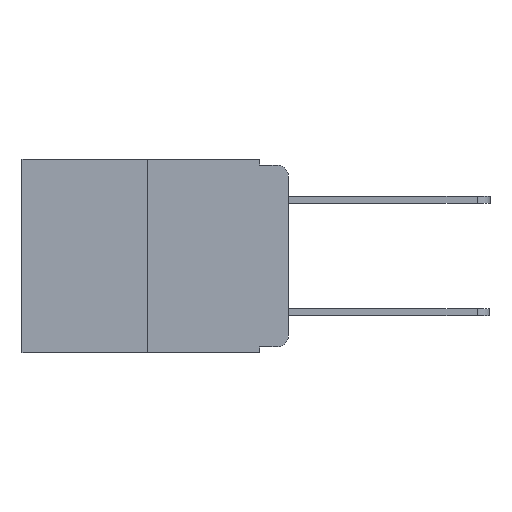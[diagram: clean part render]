
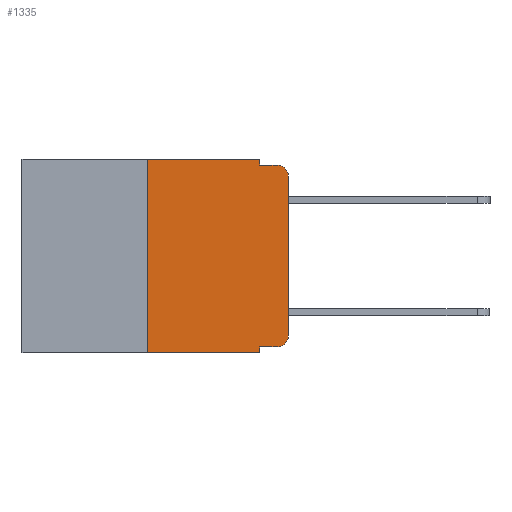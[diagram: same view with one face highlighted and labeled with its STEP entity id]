
A CAD part, left-side view. The second image highlights one B-rep face of the part: STEP entity #1335.
In plain terms, the highlighted planar face has unit normal (-1, 0, 0).
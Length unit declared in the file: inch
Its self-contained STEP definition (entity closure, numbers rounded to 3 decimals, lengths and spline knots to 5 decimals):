
#165 = VERTEX_POINT ( 'NONE', #10227 ) ;
#228 = EDGE_LOOP ( 'NONE', ( #6123, #8657, #6183, #6299, #9852, #9663, #3445, #1390, #520, #1811 ) ) ;
#249 = VECTOR ( 'NONE', #7987, 39.37008 ) ;
#341 = CARTESIAN_POINT ( 'NONE',  ( 0., 0.02, -0.01 ) ) ;
#520 = ORIENTED_EDGE ( 'NONE', *, *, #4425, .T. ) ;
#613 = FACE_OUTER_BOUND ( 'NONE', #228, .T. ) ;
#653 = EDGE_CURVE ( 'NONE', #1244, #3610, #3080, .T. ) ;
#655 = DIRECTION ( 'NONE',  ( 0., -1., 0. ) ) ;
#718 = CARTESIAN_POINT ( 'NONE',  ( 0., 0.02, -0.313 ) ) ;
#770 = VECTOR ( 'NONE', #4674, 39.37008 ) ;
#927 = VERTEX_POINT ( 'NONE', #341 ) ;
#1050 = AXIS2_PLACEMENT_3D ( 'NONE', #718, #6749, #1733 ) ;
#1244 = VERTEX_POINT ( 'NONE', #7018 ) ;
#1335 = ADVANCED_FACE ( 'NONE', ( #613 ), #2772, .F. ) ;
#1390 = ORIENTED_EDGE ( 'NONE', *, *, #4165, .F. ) ;
#1402 = VERTEX_POINT ( 'NONE', #4559 ) ;
#1494 = CARTESIAN_POINT ( 'NONE',  ( 0., 0.051, -0.343 ) ) ;
#1638 = EDGE_CURVE ( 'NONE', #5481, #4667, #7302, .T. ) ;
#1733 = DIRECTION ( 'NONE',  ( 0., 0., -1. ) ) ;
#1811 = ORIENTED_EDGE ( 'NONE', *, *, #9679, .T. ) ;
#1868 = CARTESIAN_POINT ( 'NONE',  ( 0., 0.051, 0. ) ) ;
#2772 = PLANE ( 'NONE',  #7489 ) ;
#2848 = CARTESIAN_POINT ( 'NONE',  ( 0., 0.473, 0. ) ) ;
#3031 = LINE ( 'NONE', #8495, #7039 ) ;
#3080 = LINE ( 'NONE', #7310, #6346 ) ;
#3445 = ORIENTED_EDGE ( 'NONE', *, *, #9829, .T. ) ;
#3610 = VERTEX_POINT ( 'NONE', #10456 ) ;
#3694 = CIRCLE ( 'NONE', #1050, 0.02 ) ;
#3818 = VECTOR ( 'NONE', #655, 39.37008 ) ;
#3822 = CARTESIAN_POINT ( 'NONE',  ( 0., 0.051, 0. ) ) ;
#3845 = DIRECTION ( 'NONE',  ( 0., 0., -1. ) ) ;
#4165 = EDGE_CURVE ( 'NONE', #1402, #7454, #8958, .T. ) ;
#4291 = VECTOR ( 'NONE', #4818, 39.37008 ) ;
#4425 = EDGE_CURVE ( 'NONE', #1402, #165, #6404, .T. ) ;
#4559 = CARTESIAN_POINT ( 'NONE',  ( 0., 0.051, -0.333 ) ) ;
#4602 = LINE ( 'NONE', #6904, #6456 ) ;
#4667 = VERTEX_POINT ( 'NONE', #8918 ) ;
#4674 = DIRECTION ( 'NONE',  ( 0., 0., 1. ) ) ;
#4818 = DIRECTION ( 'NONE',  ( 0., -1., 0. ) ) ;
#4907 = CARTESIAN_POINT ( 'NONE',  ( 0., 0.25, 0. ) ) ;
#5033 = DIRECTION ( 'NONE',  ( 0., 0., 1. ) ) ;
#5151 = DIRECTION ( 'NONE',  ( -1., 0., 0. ) ) ;
#5274 = VERTEX_POINT ( 'NONE', #8656 ) ;
#5403 = EDGE_CURVE ( 'NONE', #3610, #927, #7458, .T. ) ;
#5481 = VERTEX_POINT ( 'NONE', #7721 ) ;
#5763 = CARTESIAN_POINT ( 'NONE',  ( 0., 0.051, -0.01 ) ) ;
#6123 = ORIENTED_EDGE ( 'NONE', *, *, #653, .T. ) ;
#6183 = ORIENTED_EDGE ( 'NONE', *, *, #7660, .F. ) ;
#6299 = ORIENTED_EDGE ( 'NONE', *, *, #8940, .F. ) ;
#6303 = DIRECTION ( 'NONE',  ( 0., -1., 0. ) ) ;
#6346 = VECTOR ( 'NONE', #5033, 39.37008 ) ;
#6404 = LINE ( 'NONE', #7913, #4291 ) ;
#6456 = VECTOR ( 'NONE', #9105, 39.37008 ) ;
#6749 = DIRECTION ( 'NONE',  ( -1., 0., 0. ) ) ;
#6904 = CARTESIAN_POINT ( 'NONE',  ( 0., 0.473, -0.343 ) ) ;
#7014 = VECTOR ( 'NONE', #3845, 39.37008 ) ;
#7018 = CARTESIAN_POINT ( 'NONE',  ( 0., 0., -0.313 ) ) ;
#7039 = VECTOR ( 'NONE', #6303, 39.37008 ) ;
#7302 = LINE ( 'NONE', #4907, #770 ) ;
#7310 = CARTESIAN_POINT ( 'NONE',  ( 0., 0., 0. ) ) ;
#7454 = VERTEX_POINT ( 'NONE', #1494 ) ;
#7458 = CIRCLE ( 'NONE', #9370, 0.02 ) ;
#7489 = AXIS2_PLACEMENT_3D ( 'NONE', #2848, #8972, #8982 ) ;
#7660 = EDGE_CURVE ( 'NONE', #5274, #927, #7982, .T. ) ;
#7721 = CARTESIAN_POINT ( 'NONE',  ( 0., 0.25, -0.343 ) ) ;
#7913 = CARTESIAN_POINT ( 'NONE',  ( 0., 0.051, -0.333 ) ) ;
#7982 = LINE ( 'NONE', #5763, #3818 ) ;
#7987 = DIRECTION ( 'NONE',  ( 0., 0., -1. ) ) ;
#8088 = EDGE_CURVE ( 'NONE', #4667, #9719, #3031, .T. ) ;
#8238 = DIRECTION ( 'NONE',  ( 0., 0., -1. ) ) ;
#8272 = CARTESIAN_POINT ( 'NONE',  ( 0., 0.051, 0. ) ) ;
#8410 = LINE ( 'NONE', #1868, #249 ) ;
#8495 = CARTESIAN_POINT ( 'NONE',  ( 0., 0.473, 0. ) ) ;
#8656 = CARTESIAN_POINT ( 'NONE',  ( 0., 0.051, -0.01 ) ) ;
#8657 = ORIENTED_EDGE ( 'NONE', *, *, #5403, .T. ) ;
#8918 = CARTESIAN_POINT ( 'NONE',  ( 0., 0.25, 0. ) ) ;
#8940 = EDGE_CURVE ( 'NONE', #9719, #5274, #8410, .T. ) ;
#8958 = LINE ( 'NONE', #3822, #7014 ) ;
#8972 = DIRECTION ( 'NONE',  ( 1., 0., 0. ) ) ;
#8982 = DIRECTION ( 'NONE',  ( 0., 0., -1. ) ) ;
#9105 = DIRECTION ( 'NONE',  ( 0., -1., 0. ) ) ;
#9370 = AXIS2_PLACEMENT_3D ( 'NONE', #10092, #5151, #8238 ) ;
#9663 = ORIENTED_EDGE ( 'NONE', *, *, #1638, .F. ) ;
#9679 = EDGE_CURVE ( 'NONE', #165, #1244, #3694, .T. ) ;
#9719 = VERTEX_POINT ( 'NONE', #8272 ) ;
#9829 = EDGE_CURVE ( 'NONE', #5481, #7454, #4602, .T. ) ;
#9852 = ORIENTED_EDGE ( 'NONE', *, *, #8088, .F. ) ;
#10092 = CARTESIAN_POINT ( 'NONE',  ( 0., 0.02, -0.03 ) ) ;
#10227 = CARTESIAN_POINT ( 'NONE',  ( 0., 0.02, -0.333 ) ) ;
#10456 = CARTESIAN_POINT ( 'NONE',  ( 0., 0., -0.03 ) ) ;
